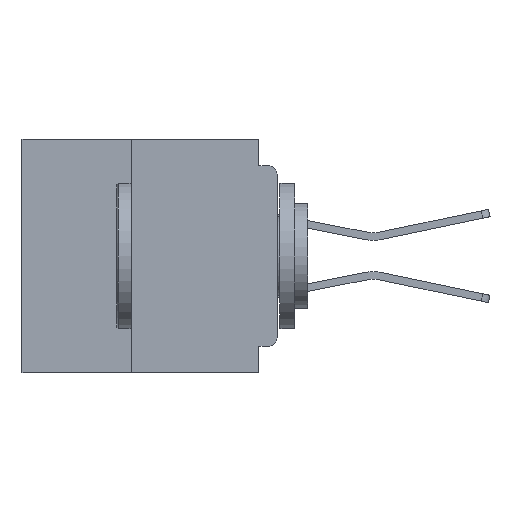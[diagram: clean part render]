
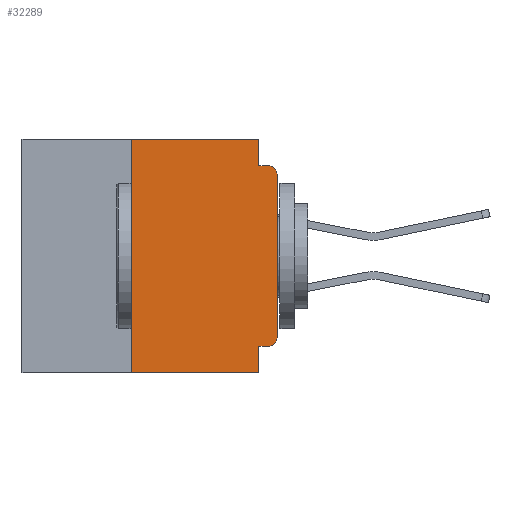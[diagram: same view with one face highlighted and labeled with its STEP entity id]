
A CAD part, left-side view. The second image highlights one B-rep face of the part: STEP entity #32289.
In plain terms, the highlighted planar face has unit normal (-1, 0, 0).
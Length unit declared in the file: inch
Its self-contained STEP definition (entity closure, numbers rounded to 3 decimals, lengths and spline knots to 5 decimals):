
#128 = VECTOR ( 'NONE', #8534, 39.37008 ) ;
#232 = LINE ( 'NONE', #22241, #1287 ) ;
#1094 = CARTESIAN_POINT ( 'NONE',  ( 0., 0.015, -0.045 ) ) ;
#1287 = VECTOR ( 'NONE', #19021, 39.37008 ) ;
#2211 = DIRECTION ( 'NONE',  ( 1., 0., 0. ) ) ;
#2461 = VECTOR ( 'NONE', #22828, 39.37008 ) ;
#2616 = DIRECTION ( 'NONE',  ( 0., 0., -1. ) ) ;
#2696 = CARTESIAN_POINT ( 'NONE',  ( 0., 0.031, 0. ) ) ;
#2815 = LINE ( 'NONE', #6343, #18827 ) ;
#3454 = LINE ( 'NONE', #19585, #2461 ) ;
#4172 = EDGE_CURVE ( 'NONE', #8925, #16403, #25835, .T. ) ;
#4303 = EDGE_CURVE ( 'NONE', #35628, #28701, #2815, .T. ) ;
#5136 = AXIS2_PLACEMENT_3D ( 'NONE', #40710, #21779, #2616 ) ;
#5250 = VECTOR ( 'NONE', #19664, 39.37008 ) ;
#5393 = CARTESIAN_POINT ( 'NONE',  ( 0., 0.015, -0.06 ) ) ;
#6202 = DIRECTION ( 'NONE',  ( 0., -1., 0. ) ) ;
#6343 = CARTESIAN_POINT ( 'NONE',  ( 0., 0.437, -0.4 ) ) ;
#6885 = AXIS2_PLACEMENT_3D ( 'NONE', #21370, #2211, #24591 ) ;
#7262 = CARTESIAN_POINT ( 'NONE',  ( 0., 0.031, -0.4 ) ) ;
#8054 = ORIENTED_EDGE ( 'NONE', *, *, #8998, .F. ) ;
#8534 = DIRECTION ( 'NONE',  ( 0., -1., 0. ) ) ;
#8634 = DIRECTION ( 'NONE',  ( 0., 0., -1. ) ) ;
#8729 = LINE ( 'NONE', #18007, #128 ) ;
#8925 = VERTEX_POINT ( 'NONE', #29124 ) ;
#8998 = EDGE_CURVE ( 'NONE', #12199, #33949, #30917, .T. ) ;
#9438 = DIRECTION ( 'NONE',  ( 0., 0., 1. ) ) ;
#9761 = CARTESIAN_POINT ( 'NONE',  ( 0., 0., 0. ) ) ;
#10494 = ORIENTED_EDGE ( 'NONE', *, *, #40609, .F. ) ;
#10800 = EDGE_CURVE ( 'NONE', #17026, #28701, #29711, .T. ) ;
#12199 = VERTEX_POINT ( 'NONE', #27400 ) ;
#12952 = FACE_OUTER_BOUND ( 'NONE', #13271, .T. ) ;
#13271 = EDGE_LOOP ( 'NONE', ( #24026, #32434, #8054, #17953, #10494, #28402, #29420, #31379, #39772, #40755 ) ) ;
#13552 = CARTESIAN_POINT ( 'NONE',  ( 0., 0., -0.045 ) ) ;
#15323 = CARTESIAN_POINT ( 'NONE',  ( 0., 0.015, -0.355 ) ) ;
#16403 = VERTEX_POINT ( 'NONE', #35573 ) ;
#17026 = VERTEX_POINT ( 'NONE', #29337 ) ;
#17953 = ORIENTED_EDGE ( 'NONE', *, *, #21511, .F. ) ;
#17991 = VECTOR ( 'NONE', #21847, 39.37008 ) ;
#18007 = CARTESIAN_POINT ( 'NONE',  ( 0., 0.437, 0. ) ) ;
#18827 = VECTOR ( 'NONE', #6202, 39.37008 ) ;
#18992 = LINE ( 'NONE', #2696, #17991 ) ;
#19021 = DIRECTION ( 'NONE',  ( 0., 1., 0. ) ) ;
#19200 = CIRCLE ( 'NONE', #5136, 0.015 ) ;
#19585 = CARTESIAN_POINT ( 'NONE',  ( 0., 0.25, -0.4 ) ) ;
#19664 = DIRECTION ( 'NONE',  ( 0., 0., -1. ) ) ;
#21222 = PLANE ( 'NONE',  #6885 ) ;
#21370 = CARTESIAN_POINT ( 'NONE',  ( 0., 0.437, 0. ) ) ;
#21511 = EDGE_CURVE ( 'NONE', #22058, #12199, #18992, .T. ) ;
#21690 = EDGE_CURVE ( 'NONE', #35628, #26753, #3454, .T. ) ;
#21779 = DIRECTION ( 'NONE',  ( -1., 0., 0. ) ) ;
#21847 = DIRECTION ( 'NONE',  ( 0., 0., -1. ) ) ;
#22058 = VERTEX_POINT ( 'NONE', #30950 ) ;
#22241 = CARTESIAN_POINT ( 'NONE',  ( 0., 0., -0.355 ) ) ;
#22494 = VECTOR ( 'NONE', #23178, 39.37008 ) ;
#22828 = DIRECTION ( 'NONE',  ( 0., 0., 1. ) ) ;
#23178 = DIRECTION ( 'NONE',  ( 0., -1., 0. ) ) ;
#23604 = CIRCLE ( 'NONE', #24913, 0.015 ) ;
#24026 = ORIENTED_EDGE ( 'NONE', *, *, #4172, .T. ) ;
#24591 = DIRECTION ( 'NONE',  ( 0., 0., -1. ) ) ;
#24913 = AXIS2_PLACEMENT_3D ( 'NONE', #5393, #27714, #8634 ) ;
#25835 = LINE ( 'NONE', #9761, #40640 ) ;
#26753 = VERTEX_POINT ( 'NONE', #39053 ) ;
#27070 = VERTEX_POINT ( 'NONE', #15323 ) ;
#27400 = CARTESIAN_POINT ( 'NONE',  ( 0., 0.031, -0.045 ) ) ;
#27714 = DIRECTION ( 'NONE',  ( -1., 0., 0. ) ) ;
#28377 = EDGE_CURVE ( 'NONE', #27070, #8925, #19200, .T. ) ;
#28402 = ORIENTED_EDGE ( 'NONE', *, *, #21690, .F. ) ;
#28701 = VERTEX_POINT ( 'NONE', #7262 ) ;
#29124 = CARTESIAN_POINT ( 'NONE',  ( 0., 0., -0.34 ) ) ;
#29337 = CARTESIAN_POINT ( 'NONE',  ( 0., 0.031, -0.355 ) ) ;
#29420 = ORIENTED_EDGE ( 'NONE', *, *, #4303, .T. ) ;
#29711 = LINE ( 'NONE', #35471, #5250 ) ;
#30917 = LINE ( 'NONE', #13552, #22494 ) ;
#30950 = CARTESIAN_POINT ( 'NONE',  ( 0., 0.031, 0. ) ) ;
#31379 = ORIENTED_EDGE ( 'NONE', *, *, #10800, .F. ) ;
#32289 = ADVANCED_FACE ( 'NONE', ( #12952 ), #21222, .F. ) ;
#32434 = ORIENTED_EDGE ( 'NONE', *, *, #36071, .T. ) ;
#33718 = EDGE_CURVE ( 'NONE', #27070, #17026, #232, .T. ) ;
#33949 = VERTEX_POINT ( 'NONE', #1094 ) ;
#35471 = CARTESIAN_POINT ( 'NONE',  ( 0., 0.031, -0.4 ) ) ;
#35573 = CARTESIAN_POINT ( 'NONE',  ( 0., 0., -0.06 ) ) ;
#35628 = VERTEX_POINT ( 'NONE', #38081 ) ;
#36071 = EDGE_CURVE ( 'NONE', #16403, #33949, #23604, .T. ) ;
#38081 = CARTESIAN_POINT ( 'NONE',  ( 0., 0.25, -0.4 ) ) ;
#39053 = CARTESIAN_POINT ( 'NONE',  ( 0., 0.25, 0. ) ) ;
#39772 = ORIENTED_EDGE ( 'NONE', *, *, #33718, .F. ) ;
#40609 = EDGE_CURVE ( 'NONE', #26753, #22058, #8729, .T. ) ;
#40640 = VECTOR ( 'NONE', #9438, 39.37008 ) ;
#40710 = CARTESIAN_POINT ( 'NONE',  ( 0., 0.015, -0.34 ) ) ;
#40755 = ORIENTED_EDGE ( 'NONE', *, *, #28377, .T. ) ;
